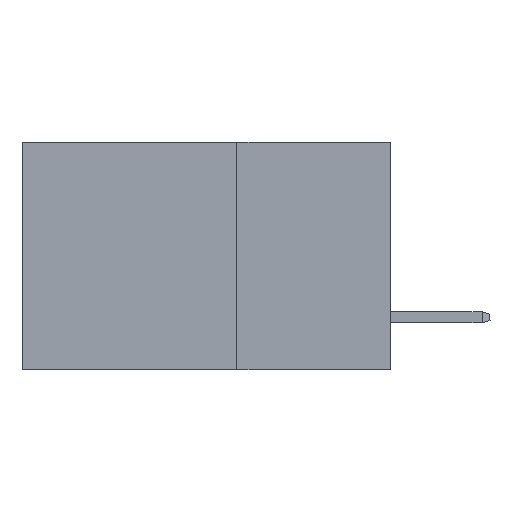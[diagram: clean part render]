
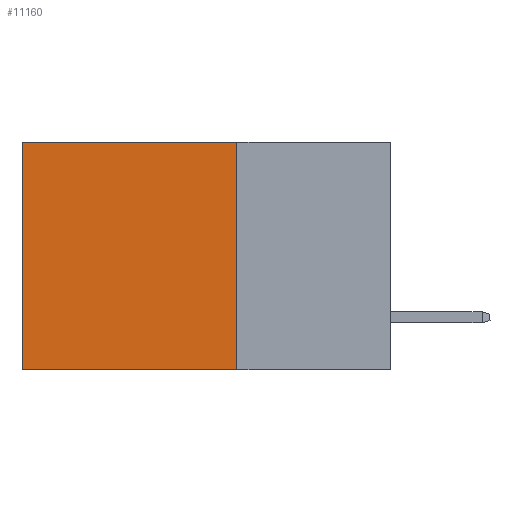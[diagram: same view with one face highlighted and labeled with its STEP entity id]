
A CAD part, left-side view. The second image highlights one B-rep face of the part: STEP entity #11160.
In plain terms, the highlighted planar face has unit normal (-1, 0, 0).
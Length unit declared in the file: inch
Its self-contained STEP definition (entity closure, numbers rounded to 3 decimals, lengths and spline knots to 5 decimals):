
#199 = ORIENTED_EDGE ( 'NONE', *, *, #13337, .F. ) ;
#203 = VECTOR ( 'NONE', #3647, 39.37008 ) ;
#379 = CARTESIAN_POINT ( 'NONE',  ( 0.2875, 0.25, -0.37 ) ) ;
#1900 = LINE ( 'NONE', #10593, #12731 ) ;
#2107 = EDGE_CURVE ( 'NONE', #4052, #13578, #3459, .T. ) ;
#3058 = ORIENTED_EDGE ( 'NONE', *, *, #2107, .T. ) ;
#3452 = ORIENTED_EDGE ( 'NONE', *, *, #4377, .F. ) ;
#3459 = LINE ( 'NONE', #5375, #203 ) ;
#3647 = DIRECTION ( 'NONE',  ( 0., 0., -1. ) ) ;
#3664 = EDGE_CURVE ( 'NONE', #7462, #4052, #1900, .T. ) ;
#3692 = VERTEX_POINT ( 'NONE', #8308 ) ;
#4052 = VERTEX_POINT ( 'NONE', #6887 ) ;
#4377 = EDGE_CURVE ( 'NONE', #7462, #3692, #5068, .T. ) ;
#4730 = AXIS2_PLACEMENT_3D ( 'NONE', #6920, #13770, #7945 ) ;
#5068 = LINE ( 'NONE', #12963, #10637 ) ;
#5375 = CARTESIAN_POINT ( 'NONE',  ( 0.2875, 0.6, 0. ) ) ;
#6519 = CARTESIAN_POINT ( 'NONE',  ( 0.2875, 0.6, -0.37 ) ) ;
#6887 = CARTESIAN_POINT ( 'NONE',  ( 0.2875, 0.6, 0. ) ) ;
#6920 = CARTESIAN_POINT ( 'NONE',  ( 0.2875, 0.25, 0. ) ) ;
#7462 = VERTEX_POINT ( 'NONE', #12875 ) ;
#7945 = DIRECTION ( 'NONE',  ( 0., 0., -1. ) ) ;
#8289 = DIRECTION ( 'NONE',  ( 0., 1., 0. ) ) ;
#8308 = CARTESIAN_POINT ( 'NONE',  ( 0.2875, 0.25, -0.37 ) ) ;
#8569 = LINE ( 'NONE', #379, #9237 ) ;
#9237 = VECTOR ( 'NONE', #8289, 39.37008 ) ;
#9319 = DIRECTION ( 'NONE',  ( 0., 1., 0. ) ) ;
#9609 = EDGE_LOOP ( 'NONE', ( #3058, #199, #3452, #11748 ) ) ;
#10593 = CARTESIAN_POINT ( 'NONE',  ( 0.2875, 0.25, 0. ) ) ;
#10637 = VECTOR ( 'NONE', #12617, 39.37008 ) ;
#10803 = FACE_OUTER_BOUND ( 'NONE', #9609, .T. ) ;
#11160 = ADVANCED_FACE ( 'NONE', ( #10803 ), #12837, .F. ) ;
#11748 = ORIENTED_EDGE ( 'NONE', *, *, #3664, .T. ) ;
#12617 = DIRECTION ( 'NONE',  ( 0., 0., -1. ) ) ;
#12731 = VECTOR ( 'NONE', #9319, 39.37008 ) ;
#12837 = PLANE ( 'NONE',  #4730 ) ;
#12875 = CARTESIAN_POINT ( 'NONE',  ( 0.2875, 0.25, 0. ) ) ;
#12963 = CARTESIAN_POINT ( 'NONE',  ( 0.2875, 0.25, 0. ) ) ;
#13337 = EDGE_CURVE ( 'NONE', #3692, #13578, #8569, .T. ) ;
#13578 = VERTEX_POINT ( 'NONE', #6519 ) ;
#13770 = DIRECTION ( 'NONE',  ( 1., 0., 0. ) ) ;
